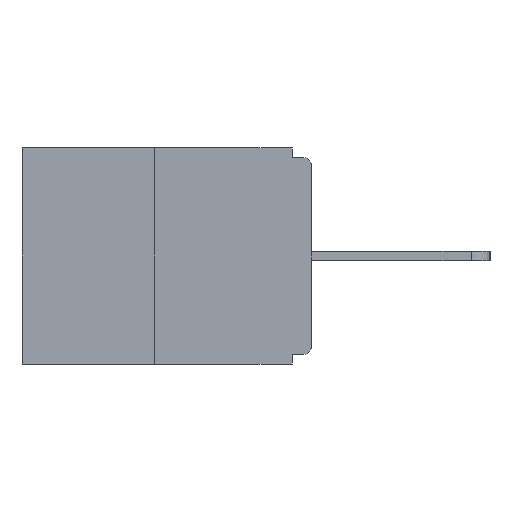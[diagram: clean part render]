
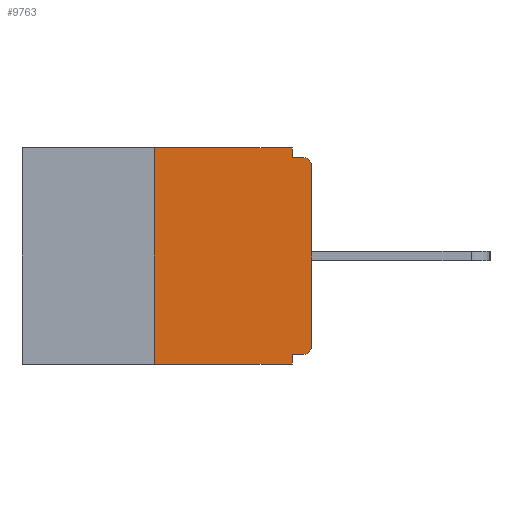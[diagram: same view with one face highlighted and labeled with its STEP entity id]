
A CAD part, left-side view. The second image highlights one B-rep face of the part: STEP entity #9763.
In plain terms, the highlighted planar face has unit normal (-1, 0, 0).
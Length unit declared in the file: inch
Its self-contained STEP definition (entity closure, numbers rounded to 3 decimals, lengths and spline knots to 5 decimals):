
#96 = DIRECTION ( 'NONE',  ( 0., -1., 0. ) ) ;
#224 = AXIS2_PLACEMENT_3D ( 'NONE', #13581, #9989, #7303 ) ;
#543 = ORIENTED_EDGE ( 'NONE', *, *, #13136, .T. ) ;
#718 = CARTESIAN_POINT ( 'NONE',  ( 0., 0.46, 0. ) ) ;
#763 = CIRCLE ( 'NONE', #10352, 0.015 ) ;
#917 = EDGE_CURVE ( 'NONE', #10695, #14940, #4966, .T. ) ;
#1273 = VERTEX_POINT ( 'NONE', #15137 ) ;
#1614 = CARTESIAN_POINT ( 'NONE',  ( 0., 0., -0.313 ) ) ;
#1644 = LINE ( 'NONE', #4212, #16408 ) ;
#1672 = VERTEX_POINT ( 'NONE', #11003 ) ;
#1806 = DIRECTION ( 'NONE',  ( 0., 0., -1. ) ) ;
#1836 = LINE ( 'NONE', #10928, #14298 ) ;
#1864 = CARTESIAN_POINT ( 'NONE',  ( 0., 0.25, 0. ) ) ;
#1969 = FACE_OUTER_BOUND ( 'NONE', #4009, .T. ) ;
#2572 = CARTESIAN_POINT ( 'NONE',  ( 0., 0., -0.03 ) ) ;
#2784 = LINE ( 'NONE', #1864, #10258 ) ;
#3216 = DIRECTION ( 'NONE',  ( 0., -1., 0. ) ) ;
#3623 = VERTEX_POINT ( 'NONE', #3881 ) ;
#3694 = EDGE_CURVE ( 'NONE', #7024, #1273, #14484, .T. ) ;
#3881 = CARTESIAN_POINT ( 'NONE',  ( 0., 0.031, -0.328 ) ) ;
#4009 = EDGE_LOOP ( 'NONE', ( #6143, #7653, #5355, #12043, #15546, #8628, #12281, #543, #12122, #10137 ) ) ;
#4212 = CARTESIAN_POINT ( 'NONE',  ( 0., 0.031, 0. ) ) ;
#4290 = DIRECTION ( 'NONE',  ( 1., 0., 0. ) ) ;
#4620 = CARTESIAN_POINT ( 'NONE',  ( 0., 0., -0.328 ) ) ;
#4689 = VECTOR ( 'NONE', #9727, 39.37008 ) ;
#4966 = CIRCLE ( 'NONE', #224, 0.015 ) ;
#5043 = CARTESIAN_POINT ( 'NONE',  ( 0., 0.031, -0.343 ) ) ;
#5226 = LINE ( 'NONE', #10005, #5320 ) ;
#5286 = DIRECTION ( 'NONE',  ( 0., 0., -1. ) ) ;
#5320 = VECTOR ( 'NONE', #96, 39.37008 ) ;
#5355 = ORIENTED_EDGE ( 'NONE', *, *, #10281, .T. ) ;
#5706 = DIRECTION ( 'NONE',  ( -1., 0., 0. ) ) ;
#5801 = CARTESIAN_POINT ( 'NONE',  ( 0., 0.015, -0.015 ) ) ;
#6143 = ORIENTED_EDGE ( 'NONE', *, *, #3694, .F. ) ;
#7024 = VERTEX_POINT ( 'NONE', #11540 ) ;
#7155 = LINE ( 'NONE', #14517, #10808 ) ;
#7156 = EDGE_CURVE ( 'NONE', #13049, #7024, #2784, .T. ) ;
#7267 = CARTESIAN_POINT ( 'NONE',  ( 0., 0.015, -0.328 ) ) ;
#7303 = DIRECTION ( 'NONE',  ( 0., 0., -1. ) ) ;
#7653 = ORIENTED_EDGE ( 'NONE', *, *, #7156, .F. ) ;
#7706 = EDGE_CURVE ( 'NONE', #3623, #14394, #7155, .T. ) ;
#7919 = LINE ( 'NONE', #9275, #10046 ) ;
#8123 = CARTESIAN_POINT ( 'NONE',  ( 0., 0.46, 0. ) ) ;
#8159 = DIRECTION ( 'NONE',  ( 0., 0., 1. ) ) ;
#8372 = EDGE_CURVE ( 'NONE', #1273, #1672, #1644, .T. ) ;
#8628 = ORIENTED_EDGE ( 'NONE', *, *, #917, .T. ) ;
#9275 = CARTESIAN_POINT ( 'NONE',  ( 0., 0., 0. ) ) ;
#9383 = EDGE_CURVE ( 'NONE', #10695, #3623, #10987, .T. ) ;
#9727 = DIRECTION ( 'NONE',  ( 0., 1., 0. ) ) ;
#9763 = ADVANCED_FACE ( 'NONE', ( #1969 ), #15730, .F. ) ;
#9989 = DIRECTION ( 'NONE',  ( -1., 0., 0. ) ) ;
#10005 = CARTESIAN_POINT ( 'NONE',  ( 0., 0., -0.015 ) ) ;
#10046 = VECTOR ( 'NONE', #8159, 39.37008 ) ;
#10137 = ORIENTED_EDGE ( 'NONE', *, *, #8372, .F. ) ;
#10258 = VECTOR ( 'NONE', #14461, 39.37008 ) ;
#10281 = EDGE_CURVE ( 'NONE', #13049, #14394, #1836, .T. ) ;
#10352 = AXIS2_PLACEMENT_3D ( 'NONE', #13402, #5706, #12148 ) ;
#10446 = VERTEX_POINT ( 'NONE', #2572 ) ;
#10695 = VERTEX_POINT ( 'NONE', #7267 ) ;
#10808 = VECTOR ( 'NONE', #12250, 39.37008 ) ;
#10928 = CARTESIAN_POINT ( 'NONE',  ( 0., 0.46, -0.343 ) ) ;
#10987 = LINE ( 'NONE', #4620, #4689 ) ;
#11003 = CARTESIAN_POINT ( 'NONE',  ( 0., 0.031, -0.015 ) ) ;
#11540 = CARTESIAN_POINT ( 'NONE',  ( 0., 0.25, 0. ) ) ;
#11827 = CARTESIAN_POINT ( 'NONE',  ( 0., 0.25, -0.343 ) ) ;
#12043 = ORIENTED_EDGE ( 'NONE', *, *, #7706, .F. ) ;
#12084 = DIRECTION ( 'NONE',  ( 0., -1., 0. ) ) ;
#12122 = ORIENTED_EDGE ( 'NONE', *, *, #15186, .F. ) ;
#12148 = DIRECTION ( 'NONE',  ( 0., 0., -1. ) ) ;
#12250 = DIRECTION ( 'NONE',  ( 0., 0., -1. ) ) ;
#12281 = ORIENTED_EDGE ( 'NONE', *, *, #12564, .T. ) ;
#12450 = VECTOR ( 'NONE', #3216, 39.37008 ) ;
#12564 = EDGE_CURVE ( 'NONE', #14940, #10446, #7919, .T. ) ;
#13049 = VERTEX_POINT ( 'NONE', #11827 ) ;
#13136 = EDGE_CURVE ( 'NONE', #10446, #14179, #763, .T. ) ;
#13402 = CARTESIAN_POINT ( 'NONE',  ( 0., 0.015, -0.03 ) ) ;
#13581 = CARTESIAN_POINT ( 'NONE',  ( 0., 0.015, -0.313 ) ) ;
#14179 = VERTEX_POINT ( 'NONE', #5801 ) ;
#14298 = VECTOR ( 'NONE', #12084, 39.37008 ) ;
#14394 = VERTEX_POINT ( 'NONE', #5043 ) ;
#14461 = DIRECTION ( 'NONE',  ( 0., 0., 1. ) ) ;
#14484 = LINE ( 'NONE', #8123, #12450 ) ;
#14517 = CARTESIAN_POINT ( 'NONE',  ( 0., 0.031, -0.343 ) ) ;
#14940 = VERTEX_POINT ( 'NONE', #1614 ) ;
#15137 = CARTESIAN_POINT ( 'NONE',  ( 0., 0.031, 0. ) ) ;
#15186 = EDGE_CURVE ( 'NONE', #1672, #14179, #5226, .T. ) ;
#15342 = AXIS2_PLACEMENT_3D ( 'NONE', #718, #4290, #1806 ) ;
#15546 = ORIENTED_EDGE ( 'NONE', *, *, #9383, .F. ) ;
#15730 = PLANE ( 'NONE',  #15342 ) ;
#16408 = VECTOR ( 'NONE', #5286, 39.37008 ) ;
